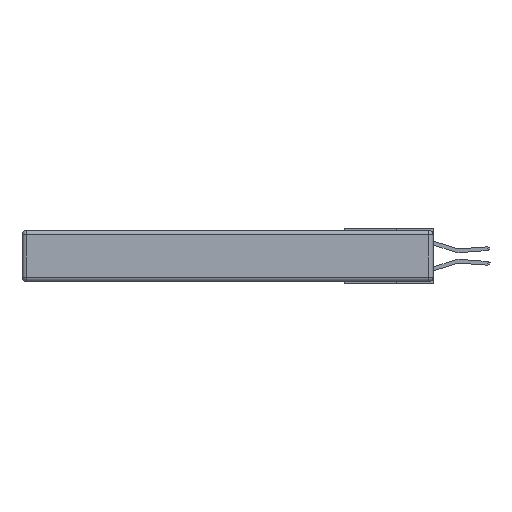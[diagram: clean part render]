
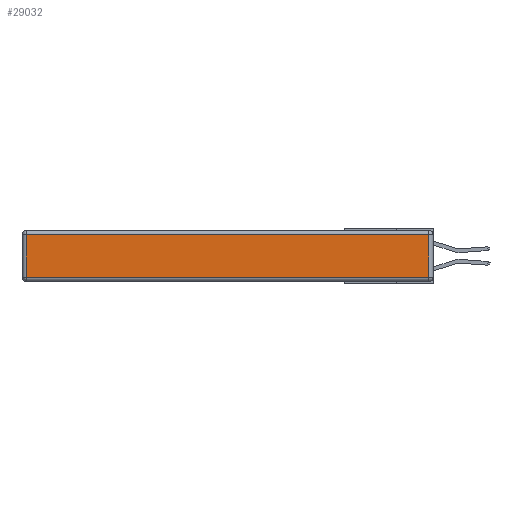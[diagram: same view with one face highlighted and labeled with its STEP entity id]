
A CAD part, left-side view. The second image highlights one B-rep face of the part: STEP entity #29032.
In plain terms, the highlighted planar face has unit normal (-1, 0, 0).
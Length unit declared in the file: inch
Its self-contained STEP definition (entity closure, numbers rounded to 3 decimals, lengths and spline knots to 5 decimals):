
#305 = ORIENTED_EDGE ( 'NONE', *, *, #27939, .T. ) ;
#765 = CARTESIAN_POINT ( 'NONE',  ( 0., 0., -0.313 ) ) ;
#1489 = DIRECTION ( 'NONE',  ( 0., 0., 1. ) ) ;
#1744 = VECTOR ( 'NONE', #1489, 39.37008 ) ;
#1968 = EDGE_CURVE ( 'NONE', #12289, #28214, #18512, .T. ) ;
#3502 = ORIENTED_EDGE ( 'NONE', *, *, #28932, .T. ) ;
#3681 = VECTOR ( 'NONE', #9199, 39.37008 ) ;
#3728 = VERTEX_POINT ( 'NONE', #13630 ) ;
#6576 = CARTESIAN_POINT ( 'NONE',  ( 0., 0., -0.343 ) ) ;
#6681 = DIRECTION ( 'NONE',  ( 0., 0., 1. ) ) ;
#7361 = FACE_OUTER_BOUND ( 'NONE', #21464, .T. ) ;
#8833 = CARTESIAN_POINT ( 'NONE',  ( 0., 2.72, -0.313 ) ) ;
#9199 = DIRECTION ( 'NONE',  ( 0., 1., 0. ) ) ;
#9868 = LINE ( 'NONE', #23156, #3681 ) ;
#12289 = VERTEX_POINT ( 'NONE', #8833 ) ;
#12721 = CARTESIAN_POINT ( 'NONE',  ( 0., 0.03, -0.313 ) ) ;
#12822 = LINE ( 'NONE', #20077, #22392 ) ;
#13630 = CARTESIAN_POINT ( 'NONE',  ( 0., 0.03, -0.03 ) ) ;
#14078 = LINE ( 'NONE', #24782, #1744 ) ;
#14786 = VECTOR ( 'NONE', #26399, 39.37008 ) ;
#16039 = AXIS2_PLACEMENT_3D ( 'NONE', #6576, #25273, #6681 ) ;
#18512 = LINE ( 'NONE', #765, #14786 ) ;
#20077 = CARTESIAN_POINT ( 'NONE',  ( 0., 2.72, -0.343 ) ) ;
#20739 = ORIENTED_EDGE ( 'NONE', *, *, #23028, .T. ) ;
#21464 = EDGE_LOOP ( 'NONE', ( #22959, #20739, #3502, #305 ) ) ;
#22037 = CARTESIAN_POINT ( 'NONE',  ( 0., 2.72, -0.03 ) ) ;
#22392 = VECTOR ( 'NONE', #22839, 39.37008 ) ;
#22839 = DIRECTION ( 'NONE',  ( 0., 0., -1. ) ) ;
#22959 = ORIENTED_EDGE ( 'NONE', *, *, #1968, .T. ) ;
#23028 = EDGE_CURVE ( 'NONE', #28214, #3728, #14078, .T. ) ;
#23044 = PLANE ( 'NONE',  #16039 ) ;
#23156 = CARTESIAN_POINT ( 'NONE',  ( 0., 2.75, -0.03 ) ) ;
#24782 = CARTESIAN_POINT ( 'NONE',  ( 0., 0.03, -0.343 ) ) ;
#25273 = DIRECTION ( 'NONE',  ( -1., 0., 0. ) ) ;
#26399 = DIRECTION ( 'NONE',  ( 0., -1., 0. ) ) ;
#27099 = VERTEX_POINT ( 'NONE', #22037 ) ;
#27939 = EDGE_CURVE ( 'NONE', #27099, #12289, #12822, .T. ) ;
#28214 = VERTEX_POINT ( 'NONE', #12721 ) ;
#28932 = EDGE_CURVE ( 'NONE', #3728, #27099, #9868, .T. ) ;
#29032 = ADVANCED_FACE ( 'NONE', ( #7361 ), #23044, .T. ) ;
